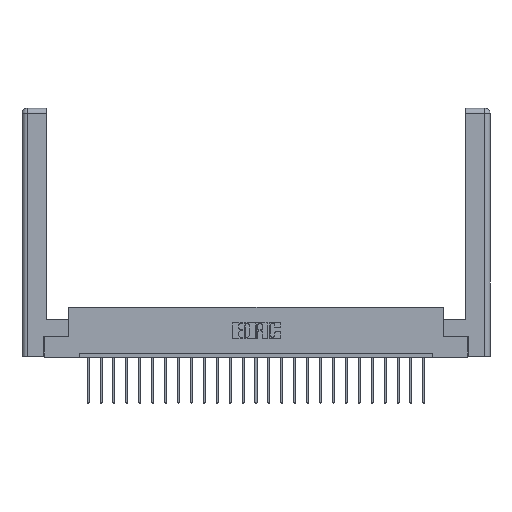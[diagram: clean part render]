
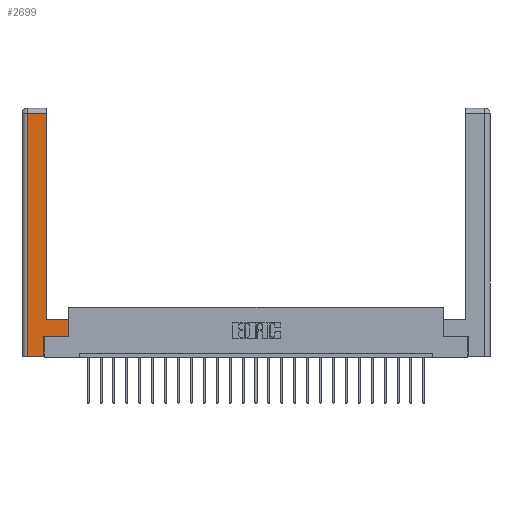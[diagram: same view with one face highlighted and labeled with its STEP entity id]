
A CAD part, top view. The second image highlights one B-rep face of the part: STEP entity #2699.
In plain terms, the highlighted planar face has unit normal (0, 0, 1).
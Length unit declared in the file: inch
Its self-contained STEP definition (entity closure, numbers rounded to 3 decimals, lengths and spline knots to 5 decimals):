
#225 = VERTEX_POINT ( 'NONE', #11941 ) ;
#423 = CARTESIAN_POINT ( 'NONE',  ( 0.295, 3., 0. ) ) ;
#635 = ORIENTED_EDGE ( 'NONE', *, *, #7974, .T. ) ;
#722 = VERTEX_POINT ( 'NONE', #5913 ) ;
#1741 = CARTESIAN_POINT ( 'NONE',  ( 0.0615, 2.94, 0. ) ) ;
#2699 = ADVANCED_FACE ( 'NONE', ( #14744 ), #5033, .F. ) ;
#2941 = VERTEX_POINT ( 'NONE', #16371 ) ;
#3251 = LINE ( 'NONE', #20120, #13043 ) ;
#3495 = AXIS2_PLACEMENT_3D ( 'NONE', #23828, #8828, #18322 ) ;
#3751 = EDGE_CURVE ( 'NONE', #22114, #722, #11104, .T. ) ;
#3936 = LINE ( 'NONE', #4584, #23878 ) ;
#4584 = CARTESIAN_POINT ( 'NONE',  ( 0.265, 0.245, 0. ) ) ;
#4839 = EDGE_CURVE ( 'NONE', #2941, #16943, #7757, .T. ) ;
#5033 = PLANE ( 'NONE',  #3495 ) ;
#5913 = CARTESIAN_POINT ( 'NONE',  ( 0.295, 0.45, 0. ) ) ;
#6117 = ORIENTED_EDGE ( 'NONE', *, *, #24188, .T. ) ;
#6195 = VECTOR ( 'NONE', #22972, 39.37008 ) ;
#6578 = LINE ( 'NONE', #423, #18698 ) ;
#7057 = LINE ( 'NONE', #1741, #6195 ) ;
#7564 = EDGE_CURVE ( 'NONE', #17070, #22621, #7057, .T. ) ;
#7757 = LINE ( 'NONE', #17306, #18780 ) ;
#7974 = EDGE_CURVE ( 'NONE', #22621, #225, #11124, .T. ) ;
#8828 = DIRECTION ( 'NONE',  ( 0., 0., -1. ) ) ;
#9231 = CARTESIAN_POINT ( 'NONE',  ( 0.265, 0., 0. ) ) ;
#9554 = CARTESIAN_POINT ( 'NONE',  ( 0.565, 0.245, 0. ) ) ;
#9577 = CARTESIAN_POINT ( 'NONE',  ( 0.295, 0.45, 0. ) ) ;
#10038 = DIRECTION ( 'NONE',  ( 1., 0., 0. ) ) ;
#10506 = VERTEX_POINT ( 'NONE', #12626 ) ;
#11104 = LINE ( 'NONE', #9577, #11370 ) ;
#11124 = LINE ( 'NONE', #20044, #11981 ) ;
#11370 = VECTOR ( 'NONE', #21338, 39.37008 ) ;
#11941 = CARTESIAN_POINT ( 'NONE',  ( 0.0615, 0., 0. ) ) ;
#11981 = VECTOR ( 'NONE', #20125, 39.37008 ) ;
#12626 = CARTESIAN_POINT ( 'NONE',  ( 0.265, 0., 0. ) ) ;
#13043 = VECTOR ( 'NONE', #22137, 39.37008 ) ;
#13409 = ORIENTED_EDGE ( 'NONE', *, *, #21137, .T. ) ;
#14101 = ORIENTED_EDGE ( 'NONE', *, *, #22064, .T. ) ;
#14744 = FACE_OUTER_BOUND ( 'NONE', #17195, .T. ) ;
#15152 = DIRECTION ( 'NONE',  ( 0., 1., 0. ) ) ;
#15646 = DIRECTION ( 'NONE',  ( 0., 1., 0. ) ) ;
#16000 = CARTESIAN_POINT ( 'NONE',  ( 0.0615, 2.94, 0. ) ) ;
#16122 = CARTESIAN_POINT ( 'NONE',  ( 0.295, 2.94, 0. ) ) ;
#16371 = CARTESIAN_POINT ( 'NONE',  ( 0.265, 0.245, 0. ) ) ;
#16943 = VERTEX_POINT ( 'NONE', #9554 ) ;
#17070 = VERTEX_POINT ( 'NONE', #16122 ) ;
#17195 = EDGE_LOOP ( 'NONE', ( #14101, #19721, #635, #6117, #13409, #17528, #20191, #18217 ) ) ;
#17306 = CARTESIAN_POINT ( 'NONE',  ( 0.565, 0.245, 0. ) ) ;
#17528 = ORIENTED_EDGE ( 'NONE', *, *, #4839, .T. ) ;
#18217 = ORIENTED_EDGE ( 'NONE', *, *, #3751, .T. ) ;
#18322 = DIRECTION ( 'NONE',  ( -1., 0., 0. ) ) ;
#18698 = VECTOR ( 'NONE', #15646, 39.37008 ) ;
#18780 = VECTOR ( 'NONE', #21152, 39.37008 ) ;
#19217 = EDGE_CURVE ( 'NONE', #16943, #22114, #3251, .T. ) ;
#19721 = ORIENTED_EDGE ( 'NONE', *, *, #7564, .T. ) ;
#19850 = VECTOR ( 'NONE', #10038, 39.37008 ) ;
#20044 = CARTESIAN_POINT ( 'NONE',  ( 0.0615, 0., 0. ) ) ;
#20120 = CARTESIAN_POINT ( 'NONE',  ( 0.565, 0.45, 0. ) ) ;
#20125 = DIRECTION ( 'NONE',  ( 0., -1., 0. ) ) ;
#20191 = ORIENTED_EDGE ( 'NONE', *, *, #19217, .T. ) ;
#20442 = LINE ( 'NONE', #9231, #19850 ) ;
#21137 = EDGE_CURVE ( 'NONE', #10506, #2941, #3936, .T. ) ;
#21152 = DIRECTION ( 'NONE',  ( 1., 0., 0. ) ) ;
#21338 = DIRECTION ( 'NONE',  ( -1., 0., 0. ) ) ;
#22064 = EDGE_CURVE ( 'NONE', #722, #17070, #6578, .T. ) ;
#22114 = VERTEX_POINT ( 'NONE', #23328 ) ;
#22137 = DIRECTION ( 'NONE',  ( 0., 1., 0. ) ) ;
#22621 = VERTEX_POINT ( 'NONE', #16000 ) ;
#22972 = DIRECTION ( 'NONE',  ( -1., 0., 0. ) ) ;
#23328 = CARTESIAN_POINT ( 'NONE',  ( 0.565, 0.45, 0. ) ) ;
#23828 = CARTESIAN_POINT ( 'NONE',  ( 0., 0., 0. ) ) ;
#23878 = VECTOR ( 'NONE', #15152, 39.37008 ) ;
#24188 = EDGE_CURVE ( 'NONE', #225, #10506, #20442, .T. ) ;
